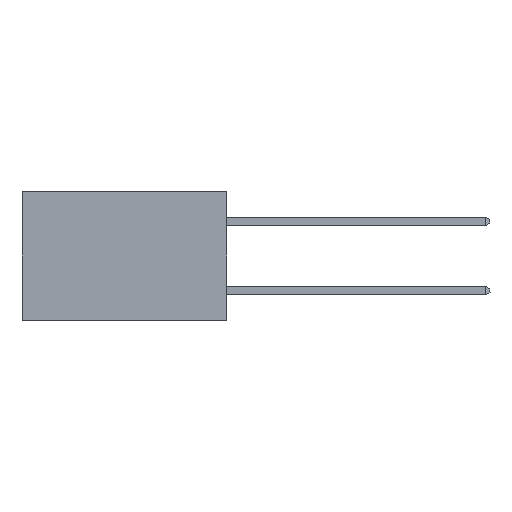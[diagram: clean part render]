
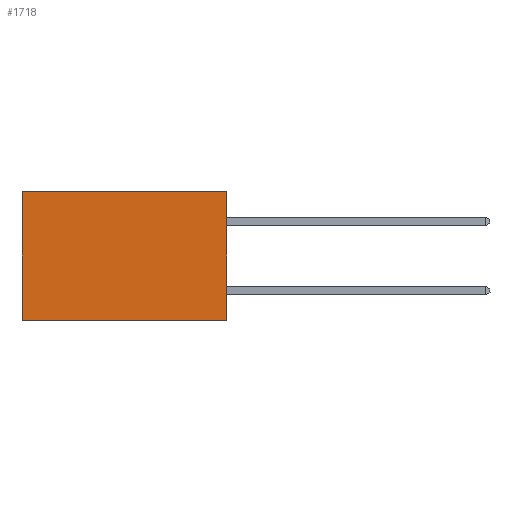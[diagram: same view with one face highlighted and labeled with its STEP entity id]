
A CAD part, left-side view. The second image highlights one B-rep face of the part: STEP entity #1718.
In plain terms, the highlighted planar face has unit normal (-1, 0, 0).
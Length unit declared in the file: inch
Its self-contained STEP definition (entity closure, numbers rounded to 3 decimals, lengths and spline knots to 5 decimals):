
#199 = VECTOR ( 'NONE', #6369, 39.37008 ) ;
#273 = EDGE_CURVE ( 'NONE', #5531, #3119, #8164, .T. ) ;
#769 = VERTEX_POINT ( 'NONE', #8315 ) ;
#824 = EDGE_LOOP ( 'NONE', ( #7730, #1347, #2214, #7296 ) ) ;
#1347 = ORIENTED_EDGE ( 'NONE', *, *, #2344, .F. ) ;
#1501 = AXIS2_PLACEMENT_3D ( 'NONE', #7856, #5824, #6608 ) ;
#1533 = CARTESIAN_POINT ( 'NONE',  ( 0.277, 0., 0. ) ) ;
#1675 = DIRECTION ( 'NONE',  ( 0., 1., 0. ) ) ;
#1718 = ADVANCED_FACE ( 'NONE', ( #6431 ), #8317, .F. ) ;
#1822 = CARTESIAN_POINT ( 'NONE',  ( 0.277, 0., 0. ) ) ;
#1887 = CARTESIAN_POINT ( 'NONE',  ( 0.277, 0.59, -0.37 ) ) ;
#2214 = ORIENTED_EDGE ( 'NONE', *, *, #273, .F. ) ;
#2344 = EDGE_CURVE ( 'NONE', #3119, #4538, #7892, .T. ) ;
#3119 = VERTEX_POINT ( 'NONE', #3290 ) ;
#3290 = CARTESIAN_POINT ( 'NONE',  ( 0.277, 0., -0.37 ) ) ;
#3398 = EDGE_CURVE ( 'NONE', #5531, #769, #6599, .T. ) ;
#4538 = VERTEX_POINT ( 'NONE', #1887 ) ;
#4646 = VECTOR ( 'NONE', #1675, 39.37008 ) ;
#4732 = VECTOR ( 'NONE', #7954, 39.37008 ) ;
#5531 = VERTEX_POINT ( 'NONE', #1822 ) ;
#5824 = DIRECTION ( 'NONE',  ( 1., 0., 0. ) ) ;
#6231 = CARTESIAN_POINT ( 'NONE',  ( 0.277, 0., -0.37 ) ) ;
#6290 = CARTESIAN_POINT ( 'NONE',  ( 0.277, 0., -0.37 ) ) ;
#6291 = EDGE_CURVE ( 'NONE', #769, #4538, #8159, .T. ) ;
#6369 = DIRECTION ( 'NONE',  ( 0., 1., 0. ) ) ;
#6431 = FACE_OUTER_BOUND ( 'NONE', #824, .T. ) ;
#6599 = LINE ( 'NONE', #1533, #4646 ) ;
#6608 = DIRECTION ( 'NONE',  ( 0., 0., -1. ) ) ;
#7296 = ORIENTED_EDGE ( 'NONE', *, *, #3398, .T. ) ;
#7730 = ORIENTED_EDGE ( 'NONE', *, *, #6291, .T. ) ;
#7856 = CARTESIAN_POINT ( 'NONE',  ( 0.277, 0., -0.37 ) ) ;
#7892 = LINE ( 'NONE', #6290, #199 ) ;
#7928 = VECTOR ( 'NONE', #8304, 39.37008 ) ;
#7954 = DIRECTION ( 'NONE',  ( 0., 0., -1. ) ) ;
#8105 = CARTESIAN_POINT ( 'NONE',  ( 0.277, 0.59, -0.37 ) ) ;
#8159 = LINE ( 'NONE', #8105, #4732 ) ;
#8164 = LINE ( 'NONE', #6231, #7928 ) ;
#8304 = DIRECTION ( 'NONE',  ( 0., 0., -1. ) ) ;
#8315 = CARTESIAN_POINT ( 'NONE',  ( 0.277, 0.59, 0. ) ) ;
#8317 = PLANE ( 'NONE',  #1501 ) ;
